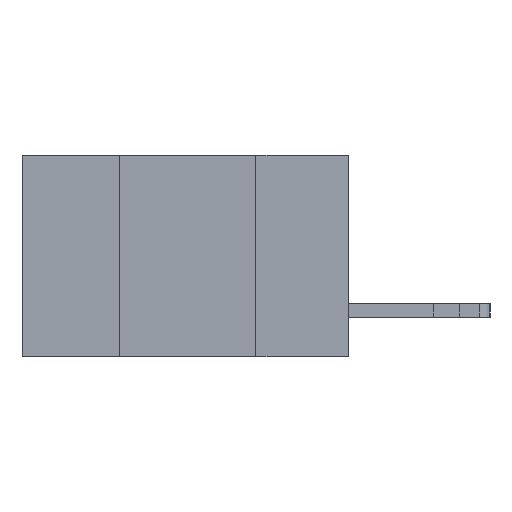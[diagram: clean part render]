
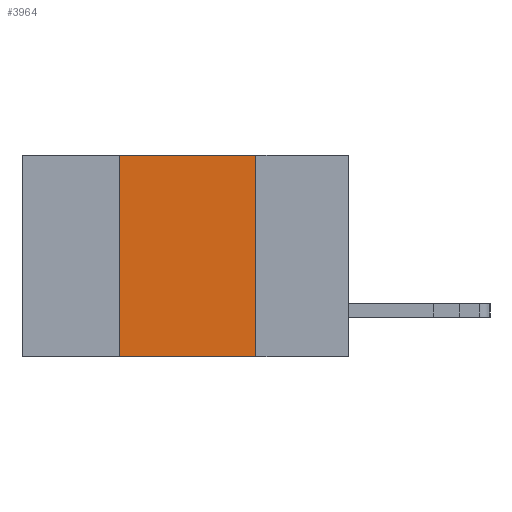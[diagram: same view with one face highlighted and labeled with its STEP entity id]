
A CAD part, left-side view. The second image highlights one B-rep face of the part: STEP entity #3964.
In plain terms, the highlighted planar face has unit normal (-1, 0, 0).
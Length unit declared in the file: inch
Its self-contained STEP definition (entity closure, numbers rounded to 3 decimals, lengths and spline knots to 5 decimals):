
#649 = CARTESIAN_POINT ( 'NONE',  ( 0., 0.42, 0. ) ) ;
#1125 = PLANE ( 'NONE',  #12682 ) ;
#2340 = CARTESIAN_POINT ( 'NONE',  ( 0., 0.6, 0. ) ) ;
#2671 = LINE ( 'NONE', #14135, #5444 ) ;
#2692 = CARTESIAN_POINT ( 'NONE',  ( 0., 0.6, 0. ) ) ;
#2859 = VERTEX_POINT ( 'NONE', #14565 ) ;
#3564 = DIRECTION ( 'NONE',  ( 1., 0., 0. ) ) ;
#3964 = ADVANCED_FACE ( 'NONE', ( #6222 ), #1125, .F. ) ;
#4241 = DIRECTION ( 'NONE',  ( 0., 0., 1. ) ) ;
#4281 = VECTOR ( 'NONE', #11753, 39.37008 ) ;
#4925 = ORIENTED_EDGE ( 'NONE', *, *, #10215, .F. ) ;
#5431 = DIRECTION ( 'NONE',  ( 0., -1., 0. ) ) ;
#5444 = VECTOR ( 'NONE', #5431, 39.37008 ) ;
#5674 = VERTEX_POINT ( 'NONE', #7492 ) ;
#5978 = VECTOR ( 'NONE', #4241, 39.37008 ) ;
#6222 = FACE_OUTER_BOUND ( 'NONE', #6893, .T. ) ;
#6540 = CARTESIAN_POINT ( 'NONE',  ( 0., 0.17, 0. ) ) ;
#6893 = EDGE_LOOP ( 'NONE', ( #13070, #7620, #4925, #10879 ) ) ;
#7028 = LINE ( 'NONE', #2692, #4281 ) ;
#7372 = VECTOR ( 'NONE', #14100, 39.37008 ) ;
#7492 = CARTESIAN_POINT ( 'NONE',  ( 0., 0.17, -0.37 ) ) ;
#7620 = ORIENTED_EDGE ( 'NONE', *, *, #7926, .F. ) ;
#7926 = EDGE_CURVE ( 'NONE', #2859, #12310, #7028, .T. ) ;
#8548 = CARTESIAN_POINT ( 'NONE',  ( 0., 0.17, 0. ) ) ;
#8903 = LINE ( 'NONE', #649, #5978 ) ;
#9479 = EDGE_CURVE ( 'NONE', #13348, #5674, #2671, .T. ) ;
#9588 = CARTESIAN_POINT ( 'NONE',  ( 0., 0.42, -0.37 ) ) ;
#10215 = EDGE_CURVE ( 'NONE', #13348, #2859, #8903, .T. ) ;
#10879 = ORIENTED_EDGE ( 'NONE', *, *, #9479, .T. ) ;
#11447 = DIRECTION ( 'NONE',  ( 0., 0., -1. ) ) ;
#11700 = EDGE_CURVE ( 'NONE', #12310, #5674, #12500, .T. ) ;
#11753 = DIRECTION ( 'NONE',  ( 0., -1., 0. ) ) ;
#12310 = VERTEX_POINT ( 'NONE', #8548 ) ;
#12500 = LINE ( 'NONE', #6540, #7372 ) ;
#12682 = AXIS2_PLACEMENT_3D ( 'NONE', #2340, #3564, #11447 ) ;
#13070 = ORIENTED_EDGE ( 'NONE', *, *, #11700, .F. ) ;
#13348 = VERTEX_POINT ( 'NONE', #9588 ) ;
#14100 = DIRECTION ( 'NONE',  ( 0., 0., -1. ) ) ;
#14135 = CARTESIAN_POINT ( 'NONE',  ( 0., 0.6, -0.37 ) ) ;
#14565 = CARTESIAN_POINT ( 'NONE',  ( 0., 0.42, 0. ) ) ;
